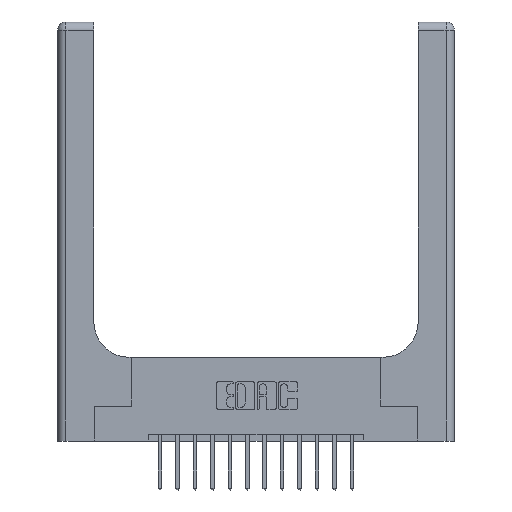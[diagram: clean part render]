
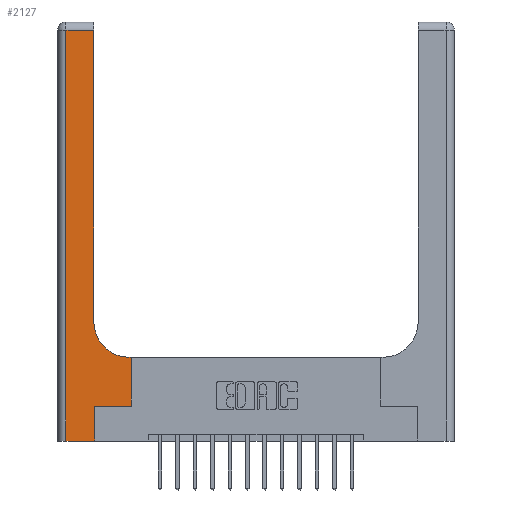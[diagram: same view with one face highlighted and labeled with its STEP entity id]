
A CAD part, top view. The second image highlights one B-rep face of the part: STEP entity #2127.
In plain terms, the highlighted planar face has unit normal (0, 0, 1).
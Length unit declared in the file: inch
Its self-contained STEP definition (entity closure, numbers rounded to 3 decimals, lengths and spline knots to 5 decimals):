
#64 = CARTESIAN_POINT ( 'NONE',  ( 0.06, 3., 0.37 ) ) ;
#675 = ORIENTED_EDGE ( 'NONE', *, *, #3472, .T. ) ;
#941 = ORIENTED_EDGE ( 'NONE', *, *, #12260, .T. ) ;
#1138 = ORIENTED_EDGE ( 'NONE', *, *, #8186, .T. ) ;
#1163 = LINE ( 'NONE', #15773, #7935 ) ;
#2127 = ADVANCED_FACE ( 'NONE', ( #6069 ), #8640, .F. ) ;
#2142 = CARTESIAN_POINT ( 'NONE',  ( 0.51, 0.6, 0.37 ) ) ;
#2154 = CARTESIAN_POINT ( 'NONE',  ( 0.265, 0.25, 0.37 ) ) ;
#2237 = LINE ( 'NONE', #7661, #17247 ) ;
#2408 = VECTOR ( 'NONE', #3837, 39.37008 ) ;
#2499 = VERTEX_POINT ( 'NONE', #12716 ) ;
#2809 = ORIENTED_EDGE ( 'NONE', *, *, #4683, .T. ) ;
#2839 = ORIENTED_EDGE ( 'NONE', *, *, #14564, .T. ) ;
#3012 = VECTOR ( 'NONE', #6534, 39.37008 ) ;
#3472 = EDGE_CURVE ( 'NONE', #12626, #11067, #17112, .T. ) ;
#3837 = DIRECTION ( 'NONE',  ( 1., 0., 0. ) ) ;
#4213 = ORIENTED_EDGE ( 'NONE', *, *, #16554, .T. ) ;
#4237 = CARTESIAN_POINT ( 'NONE',  ( 0.51, 0.85, 0.37 ) ) ;
#4412 = LINE ( 'NONE', #9793, #15710 ) ;
#4554 = CARTESIAN_POINT ( 'NONE',  ( 0.26, 2.94, 0.37 ) ) ;
#4622 = VERTEX_POINT ( 'NONE', #15635 ) ;
#4674 = DIRECTION ( 'NONE',  ( 0., 0., -1. ) ) ;
#4683 = EDGE_CURVE ( 'NONE', #11067, #14119, #5130, .T. ) ;
#5130 = LINE ( 'NONE', #17147, #3012 ) ;
#5551 = ORIENTED_EDGE ( 'NONE', *, *, #8180, .T. ) ;
#6069 = FACE_OUTER_BOUND ( 'NONE', #6077, .T. ) ;
#6077 = EDGE_LOOP ( 'NONE', ( #5551, #8743, #2839, #1138, #4213, #675, #2809, #941, #15215 ) ) ;
#6534 = DIRECTION ( 'NONE',  ( 0., 1., 0. ) ) ;
#6910 = CARTESIAN_POINT ( 'NONE',  ( 0.528, 0.25, 0.37 ) ) ;
#7633 = VECTOR ( 'NONE', #10285, 39.37008 ) ;
#7661 = CARTESIAN_POINT ( 'NONE',  ( 0.26, 3., 0.37 ) ) ;
#7921 = LINE ( 'NONE', #13282, #7633 ) ;
#7935 = VECTOR ( 'NONE', #11944, 39.37008 ) ;
#8007 = CARTESIAN_POINT ( 'NONE',  ( 0.06, 0., 0.37 ) ) ;
#8050 = EDGE_CURVE ( 'NONE', #9563, #10436, #7921, .T. ) ;
#8180 = EDGE_CURVE ( 'NONE', #2499, #9563, #2237, .T. ) ;
#8186 = EDGE_CURVE ( 'NONE', #17065, #4622, #1163, .T. ) ;
#8214 = DIRECTION ( 'NONE',  ( 0., 0., -1. ) ) ;
#8474 = EDGE_CURVE ( 'NONE', #10369, #2499, #16285, .T. ) ;
#8640 = PLANE ( 'NONE',  #14493 ) ;
#8743 = ORIENTED_EDGE ( 'NONE', *, *, #8050, .T. ) ;
#9232 = DIRECTION ( 'NONE',  ( 0., 1., 0. ) ) ;
#9563 = VERTEX_POINT ( 'NONE', #4554 ) ;
#9793 = CARTESIAN_POINT ( 'NONE',  ( 0.26, 0.6, 0.37 ) ) ;
#10034 = DIRECTION ( 'NONE',  ( -1., 0., 0. ) ) ;
#10285 = DIRECTION ( 'NONE',  ( -1., 0., 0. ) ) ;
#10369 = VERTEX_POINT ( 'NONE', #2142 ) ;
#10436 = VERTEX_POINT ( 'NONE', #15587 ) ;
#10490 = CARTESIAN_POINT ( 'NONE',  ( 0.265, 0., 0.37 ) ) ;
#10548 = CARTESIAN_POINT ( 'NONE',  ( 0.265, 0.25, 0.37 ) ) ;
#10655 = DIRECTION ( 'NONE',  ( 0., 1., 0. ) ) ;
#11067 = VERTEX_POINT ( 'NONE', #6910 ) ;
#11353 = CARTESIAN_POINT ( 'NONE',  ( 0., 3., 0.37 ) ) ;
#11944 = DIRECTION ( 'NONE',  ( 1., 0., 0. ) ) ;
#12182 = LINE ( 'NONE', #64, #14694 ) ;
#12260 = EDGE_CURVE ( 'NONE', #14119, #10369, #4412, .T. ) ;
#12582 = AXIS2_PLACEMENT_3D ( 'NONE', #4237, #8214, #14993 ) ;
#12626 = VERTEX_POINT ( 'NONE', #10548 ) ;
#12716 = CARTESIAN_POINT ( 'NONE',  ( 0.26, 0.85, 0.37 ) ) ;
#12848 = VECTOR ( 'NONE', #10655, 39.37008 ) ;
#13282 = CARTESIAN_POINT ( 'NONE',  ( 0., 2.94, 0.37 ) ) ;
#14119 = VERTEX_POINT ( 'NONE', #14682 ) ;
#14493 = AXIS2_PLACEMENT_3D ( 'NONE', #11353, #4674, #10034 ) ;
#14564 = EDGE_CURVE ( 'NONE', #10436, #17065, #12182, .T. ) ;
#14682 = CARTESIAN_POINT ( 'NONE',  ( 0.528, 0.6, 0.37 ) ) ;
#14694 = VECTOR ( 'NONE', #16269, 39.37008 ) ;
#14993 = DIRECTION ( 'NONE',  ( 1., 0., 0. ) ) ;
#15215 = ORIENTED_EDGE ( 'NONE', *, *, #8474, .T. ) ;
#15587 = CARTESIAN_POINT ( 'NONE',  ( 0.06, 2.94, 0.37 ) ) ;
#15635 = CARTESIAN_POINT ( 'NONE',  ( 0.265, 0., 0.37 ) ) ;
#15710 = VECTOR ( 'NONE', #16689, 39.37008 ) ;
#15773 = CARTESIAN_POINT ( 'NONE',  ( 0., 0., 0.37 ) ) ;
#16269 = DIRECTION ( 'NONE',  ( 0., -1., 0. ) ) ;
#16285 = CIRCLE ( 'NONE', #12582, 0.25 ) ;
#16554 = EDGE_CURVE ( 'NONE', #4622, #12626, #17232, .T. ) ;
#16689 = DIRECTION ( 'NONE',  ( -1., 0., 0. ) ) ;
#17065 = VERTEX_POINT ( 'NONE', #8007 ) ;
#17112 = LINE ( 'NONE', #2154, #2408 ) ;
#17147 = CARTESIAN_POINT ( 'NONE',  ( 0.528, 0.25, 0.37 ) ) ;
#17232 = LINE ( 'NONE', #10490, #12848 ) ;
#17247 = VECTOR ( 'NONE', #9232, 39.37008 ) ;
